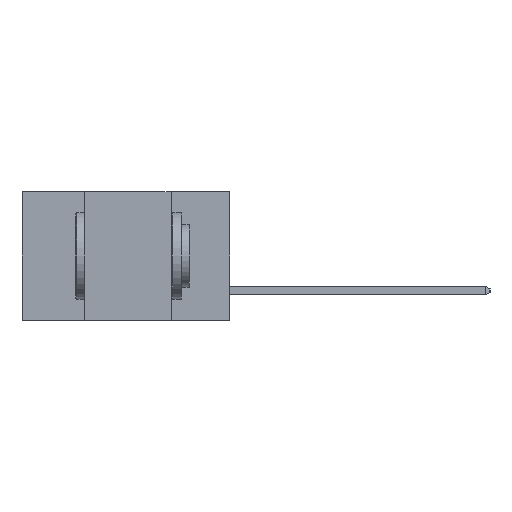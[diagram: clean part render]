
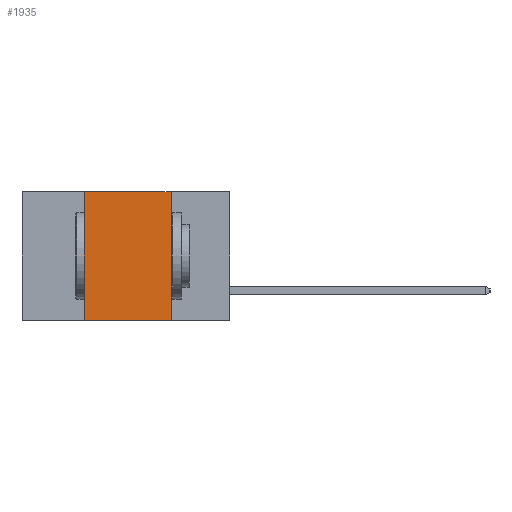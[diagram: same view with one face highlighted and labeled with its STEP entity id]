
A CAD part, left-side view. The second image highlights one B-rep face of the part: STEP entity #1935.
In plain terms, the highlighted planar face has unit normal (-1, 0, 0).
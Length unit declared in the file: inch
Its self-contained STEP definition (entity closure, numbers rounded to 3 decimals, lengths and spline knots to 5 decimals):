
#213 = CARTESIAN_POINT ( 'NONE',  ( 0., 0.6, 0. ) ) ;
#389 = DIRECTION ( 'NONE',  ( 0., -1., 0. ) ) ;
#702 = LINE ( 'NONE', #7830, #7716 ) ;
#708 = VERTEX_POINT ( 'NONE', #3735 ) ;
#719 = VERTEX_POINT ( 'NONE', #1272 ) ;
#877 = EDGE_CURVE ( 'NONE', #719, #708, #3823, .T. ) ;
#894 = DIRECTION ( 'NONE',  ( 0., 0., -1. ) ) ;
#941 = DIRECTION ( 'NONE',  ( 1., 0., 0. ) ) ;
#1105 = VERTEX_POINT ( 'NONE', #8602 ) ;
#1272 = CARTESIAN_POINT ( 'NONE',  ( 0., 0.42, -0.37 ) ) ;
#1526 = CARTESIAN_POINT ( 'NONE',  ( 0., 0.42, -0.37 ) ) ;
#1593 = VERTEX_POINT ( 'NONE', #3180 ) ;
#1935 = ADVANCED_FACE ( 'NONE', ( #2275 ), #7064, .F. ) ;
#1997 = ORIENTED_EDGE ( 'NONE', *, *, #2774, .F. ) ;
#2275 = FACE_OUTER_BOUND ( 'NONE', #10503, .T. ) ;
#2774 = EDGE_CURVE ( 'NONE', #719, #1593, #10393, .T. ) ;
#3180 = CARTESIAN_POINT ( 'NONE',  ( 0., 0.42, 0. ) ) ;
#3343 = DIRECTION ( 'NONE',  ( 0., 0., 1. ) ) ;
#3735 = CARTESIAN_POINT ( 'NONE',  ( 0., 0.17, -0.37 ) ) ;
#3823 = LINE ( 'NONE', #7099, #5769 ) ;
#4558 = ORIENTED_EDGE ( 'NONE', *, *, #877, .T. ) ;
#4738 = EDGE_CURVE ( 'NONE', #1593, #1105, #9296, .T. ) ;
#5382 = EDGE_CURVE ( 'NONE', #1105, #708, #702, .T. ) ;
#5769 = VECTOR ( 'NONE', #7156, 39.37008 ) ;
#5999 = VECTOR ( 'NONE', #3343, 39.37008 ) ;
#7037 = CARTESIAN_POINT ( 'NONE',  ( 0., 0.6, 0. ) ) ;
#7064 = PLANE ( 'NONE',  #8471 ) ;
#7099 = CARTESIAN_POINT ( 'NONE',  ( 0., 0.6, -0.37 ) ) ;
#7104 = VECTOR ( 'NONE', #389, 39.37008 ) ;
#7156 = DIRECTION ( 'NONE',  ( 0., -1., 0. ) ) ;
#7716 = VECTOR ( 'NONE', #7803, 39.37008 ) ;
#7803 = DIRECTION ( 'NONE',  ( 0., 0., -1. ) ) ;
#7830 = CARTESIAN_POINT ( 'NONE',  ( 0., 0.17, -0.37 ) ) ;
#8280 = ORIENTED_EDGE ( 'NONE', *, *, #5382, .F. ) ;
#8471 = AXIS2_PLACEMENT_3D ( 'NONE', #7037, #941, #894 ) ;
#8533 = ORIENTED_EDGE ( 'NONE', *, *, #4738, .F. ) ;
#8602 = CARTESIAN_POINT ( 'NONE',  ( 0., 0.17, 0. ) ) ;
#9296 = LINE ( 'NONE', #213, #7104 ) ;
#10393 = LINE ( 'NONE', #1526, #5999 ) ;
#10503 = EDGE_LOOP ( 'NONE', ( #8280, #8533, #1997, #4558 ) ) ;
